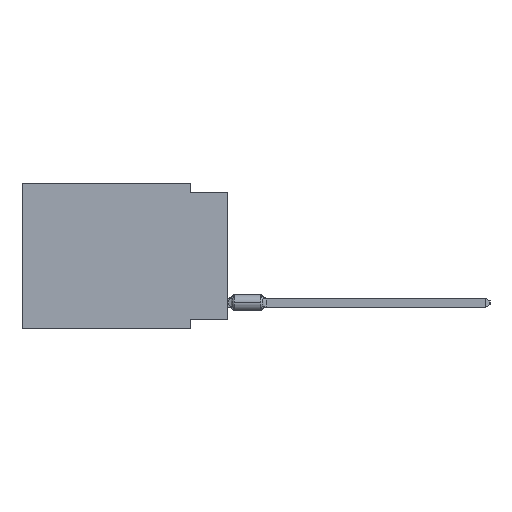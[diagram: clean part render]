
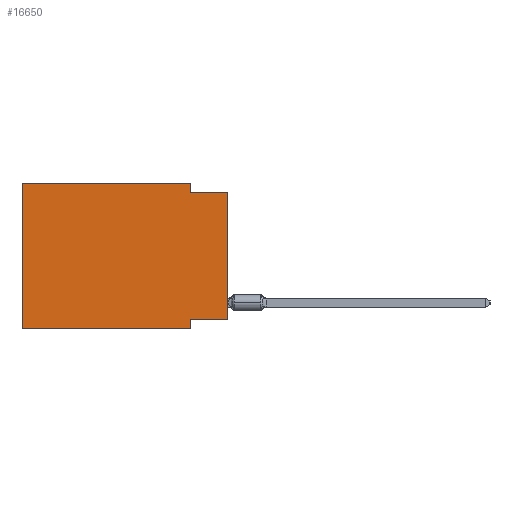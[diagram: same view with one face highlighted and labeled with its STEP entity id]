
A CAD part, left-side view. The second image highlights one B-rep face of the part: STEP entity #16650.
In plain terms, the highlighted planar face has unit normal (-1, 0, 0).
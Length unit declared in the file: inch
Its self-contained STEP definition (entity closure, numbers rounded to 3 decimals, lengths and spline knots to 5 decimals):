
#2175 = VERTEX_POINT ( 'NONE', #51583 ) ;
#4186 = ORIENTED_EDGE ( 'NONE', *, *, #57994, .F. ) ;
#4285 = DIRECTION ( 'NONE',  ( 1., 0., 0. ) ) ;
#5444 = DIRECTION ( 'NONE',  ( 0., 0., -1. ) ) ;
#6226 = DIRECTION ( 'NONE',  ( 0., 1., 0. ) ) ;
#9203 = LINE ( 'NONE', #31759, #26051 ) ;
#9331 = CARTESIAN_POINT ( 'NONE',  ( 0., 0.55, 0. ) ) ;
#9587 = EDGE_CURVE ( 'NONE', #35164, #43147, #27306, .T. ) ;
#10377 = ORIENTED_EDGE ( 'NONE', *, *, #38537, .F. ) ;
#10881 = ORIENTED_EDGE ( 'NONE', *, *, #41218, .F. ) ;
#11948 = EDGE_CURVE ( 'NONE', #30380, #53172, #32887, .T. ) ;
#12754 = LINE ( 'NONE', #25656, #49568 ) ;
#14450 = CARTESIAN_POINT ( 'NONE',  ( 0., 0.55, -0.39 ) ) ;
#16650 = ADVANCED_FACE ( 'NONE', ( #27698 ), #53808, .F. ) ;
#17503 = EDGE_LOOP ( 'NONE', ( #54975, #4186, #43907, #47958, #10377, #44683, #10881, #46565 ) ) ;
#17954 = VERTEX_POINT ( 'NONE', #9331 ) ;
#18825 = LINE ( 'NONE', #44608, #21201 ) ;
#19574 = EDGE_CURVE ( 'NONE', #17954, #35164, #37277, .T. ) ;
#21201 = VECTOR ( 'NONE', #54294, 39.37008 ) ;
#21417 = CARTESIAN_POINT ( 'NONE',  ( 0., 0., 0. ) ) ;
#21834 = DIRECTION ( 'NONE',  ( 0., 0., -1. ) ) ;
#22954 = DIRECTION ( 'NONE',  ( 0., -1., 0. ) ) ;
#25656 = CARTESIAN_POINT ( 'NONE',  ( 0., 0.1, -0.39 ) ) ;
#26026 = EDGE_CURVE ( 'NONE', #30380, #49361, #48067, .T. ) ;
#26051 = VECTOR ( 'NONE', #41113, 39.37008 ) ;
#27020 = DIRECTION ( 'NONE',  ( 0., 0., -1. ) ) ;
#27306 = LINE ( 'NONE', #44309, #53614 ) ;
#27698 = FACE_OUTER_BOUND ( 'NONE', #17503, .T. ) ;
#28428 = LINE ( 'NONE', #29293, #53264 ) ;
#29293 = CARTESIAN_POINT ( 'NONE',  ( 0., 0.55, -0.39 ) ) ;
#30380 = VERTEX_POINT ( 'NONE', #46160 ) ;
#31759 = CARTESIAN_POINT ( 'NONE',  ( 0., 0.55, 0. ) ) ;
#32887 = LINE ( 'NONE', #55194, #45345 ) ;
#33187 = AXIS2_PLACEMENT_3D ( 'NONE', #45566, #4285, #5444 ) ;
#33682 = DIRECTION ( 'NONE',  ( 0., -1., 0. ) ) ;
#35164 = VERTEX_POINT ( 'NONE', #56269 ) ;
#37006 = EDGE_CURVE ( 'NONE', #50223, #2175, #28428, .T. ) ;
#37277 = LINE ( 'NONE', #45797, #44629 ) ;
#38537 = EDGE_CURVE ( 'NONE', #50223, #17954, #9203, .T. ) ;
#39271 = DIRECTION ( 'NONE',  ( 0., 0., 1. ) ) ;
#40767 = CARTESIAN_POINT ( 'NONE',  ( 0., 0.1, -0.025 ) ) ;
#41113 = DIRECTION ( 'NONE',  ( 0., 0., 1. ) ) ;
#41218 = EDGE_CURVE ( 'NONE', #53172, #2175, #12754, .T. ) ;
#42830 = CARTESIAN_POINT ( 'NONE',  ( 0., 0., -0.025 ) ) ;
#43147 = VERTEX_POINT ( 'NONE', #40767 ) ;
#43907 = ORIENTED_EDGE ( 'NONE', *, *, #9587, .F. ) ;
#44309 = CARTESIAN_POINT ( 'NONE',  ( 0., 0.1, 0. ) ) ;
#44608 = CARTESIAN_POINT ( 'NONE',  ( 0., 0., -0.025 ) ) ;
#44629 = VECTOR ( 'NONE', #22954, 39.37008 ) ;
#44683 = ORIENTED_EDGE ( 'NONE', *, *, #37006, .T. ) ;
#45345 = VECTOR ( 'NONE', #6226, 39.37008 ) ;
#45566 = CARTESIAN_POINT ( 'NONE',  ( 0., 0.55, 0. ) ) ;
#45797 = CARTESIAN_POINT ( 'NONE',  ( 0., 0.55, 0. ) ) ;
#46160 = CARTESIAN_POINT ( 'NONE',  ( 0., 0., -0.365 ) ) ;
#46565 = ORIENTED_EDGE ( 'NONE', *, *, #11948, .F. ) ;
#47958 = ORIENTED_EDGE ( 'NONE', *, *, #19574, .F. ) ;
#48067 = LINE ( 'NONE', #21417, #51555 ) ;
#49361 = VERTEX_POINT ( 'NONE', #42830 ) ;
#49568 = VECTOR ( 'NONE', #21834, 39.37008 ) ;
#50223 = VERTEX_POINT ( 'NONE', #14450 ) ;
#51555 = VECTOR ( 'NONE', #39271, 39.37008 ) ;
#51583 = CARTESIAN_POINT ( 'NONE',  ( 0., 0.1, -0.39 ) ) ;
#53172 = VERTEX_POINT ( 'NONE', #55054 ) ;
#53264 = VECTOR ( 'NONE', #33682, 39.37008 ) ;
#53614 = VECTOR ( 'NONE', #27020, 39.37008 ) ;
#53808 = PLANE ( 'NONE',  #33187 ) ;
#54294 = DIRECTION ( 'NONE',  ( 0., -1., 0. ) ) ;
#54975 = ORIENTED_EDGE ( 'NONE', *, *, #26026, .T. ) ;
#55054 = CARTESIAN_POINT ( 'NONE',  ( 0., 0.1, -0.365 ) ) ;
#55194 = CARTESIAN_POINT ( 'NONE',  ( 0., 0., -0.365 ) ) ;
#56269 = CARTESIAN_POINT ( 'NONE',  ( 0., 0.1, 0. ) ) ;
#57994 = EDGE_CURVE ( 'NONE', #43147, #49361, #18825, .T. ) ;
